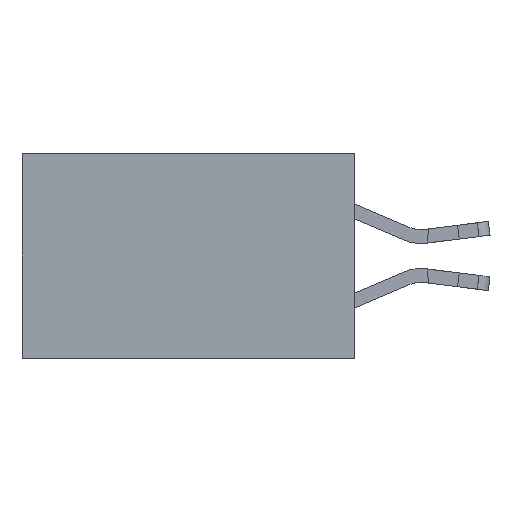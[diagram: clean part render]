
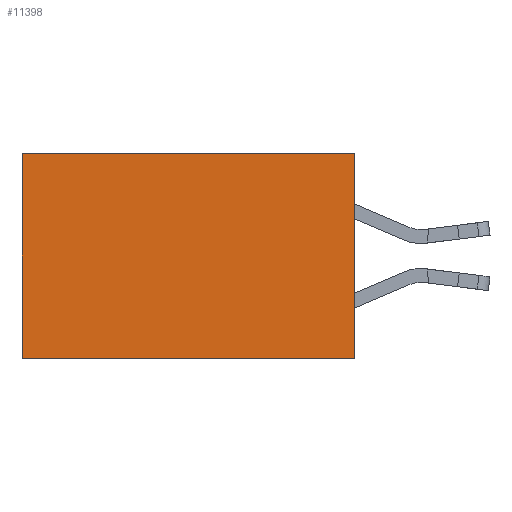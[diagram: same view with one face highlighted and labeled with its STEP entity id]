
A CAD part, left-side view. The second image highlights one B-rep face of the part: STEP entity #11398.
In plain terms, the highlighted planar face has unit normal (-1, 0, 0).
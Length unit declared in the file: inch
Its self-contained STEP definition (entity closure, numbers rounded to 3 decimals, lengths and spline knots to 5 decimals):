
#302 = CARTESIAN_POINT ( 'NONE',  ( 0.298, 0.6, 0. ) ) ;
#951 = VECTOR ( 'NONE', #11824, 39.37008 ) ;
#1040 = VECTOR ( 'NONE', #17891, 39.37008 ) ;
#1230 = AXIS2_PLACEMENT_3D ( 'NONE', #4104, #5603, #15904 ) ;
#1782 = EDGE_LOOP ( 'NONE', ( #16852, #12104, #12923, #13098 ) ) ;
#2606 = PLANE ( 'NONE',  #1230 ) ;
#3038 = VERTEX_POINT ( 'NONE', #13359 ) ;
#3131 = VECTOR ( 'NONE', #8196, 39.37008 ) ;
#4070 = VERTEX_POINT ( 'NONE', #11976 ) ;
#4104 = CARTESIAN_POINT ( 'NONE',  ( 0.298, 0., 0. ) ) ;
#4788 = CARTESIAN_POINT ( 'NONE',  ( 0.298, 0., -0.37 ) ) ;
#5603 = DIRECTION ( 'NONE',  ( 1., 0., 0. ) ) ;
#6843 = LINE ( 'NONE', #302, #18031 ) ;
#7713 = CARTESIAN_POINT ( 'NONE',  ( 0.298, 0., 0. ) ) ;
#8196 = DIRECTION ( 'NONE',  ( 0., 1., 0. ) ) ;
#10370 = CARTESIAN_POINT ( 'NONE',  ( 0.298, 0., 0. ) ) ;
#10997 = EDGE_CURVE ( 'NONE', #3038, #4070, #6843, .T. ) ;
#11153 = CARTESIAN_POINT ( 'NONE',  ( 0.298, 0., -0.37 ) ) ;
#11398 = ADVANCED_FACE ( 'NONE', ( #12135 ), #2606, .F. ) ;
#11535 = EDGE_CURVE ( 'NONE', #16535, #3038, #12831, .T. ) ;
#11824 = DIRECTION ( 'NONE',  ( 0., 1., 0. ) ) ;
#11976 = CARTESIAN_POINT ( 'NONE',  ( 0.298, 0.6, -0.37 ) ) ;
#12104 = ORIENTED_EDGE ( 'NONE', *, *, #15722, .F. ) ;
#12135 = FACE_OUTER_BOUND ( 'NONE', #1782, .T. ) ;
#12155 = DIRECTION ( 'NONE',  ( 0., 0., -1. ) ) ;
#12455 = LINE ( 'NONE', #7713, #1040 ) ;
#12831 = LINE ( 'NONE', #10370, #951 ) ;
#12923 = ORIENTED_EDGE ( 'NONE', *, *, #14788, .F. ) ;
#13098 = ORIENTED_EDGE ( 'NONE', *, *, #11535, .T. ) ;
#13359 = CARTESIAN_POINT ( 'NONE',  ( 0.298, 0.6, 0. ) ) ;
#14501 = LINE ( 'NONE', #11153, #3131 ) ;
#14788 = EDGE_CURVE ( 'NONE', #16535, #14864, #12455, .T. ) ;
#14864 = VERTEX_POINT ( 'NONE', #4788 ) ;
#15000 = CARTESIAN_POINT ( 'NONE',  ( 0.298, 0., 0. ) ) ;
#15722 = EDGE_CURVE ( 'NONE', #14864, #4070, #14501, .T. ) ;
#15904 = DIRECTION ( 'NONE',  ( 0., 0., -1. ) ) ;
#16535 = VERTEX_POINT ( 'NONE', #15000 ) ;
#16852 = ORIENTED_EDGE ( 'NONE', *, *, #10997, .T. ) ;
#17891 = DIRECTION ( 'NONE',  ( 0., 0., -1. ) ) ;
#18031 = VECTOR ( 'NONE', #12155, 39.37008 ) ;
